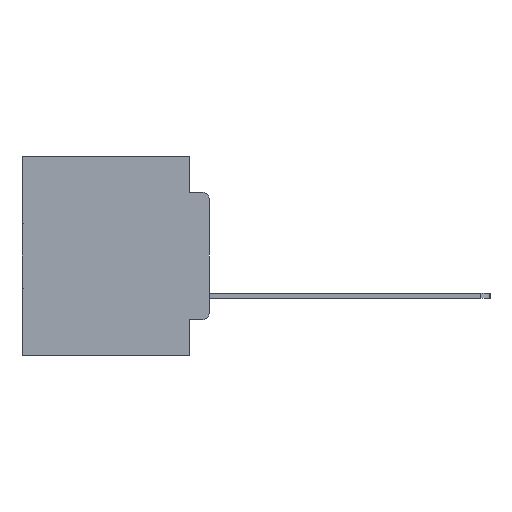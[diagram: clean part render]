
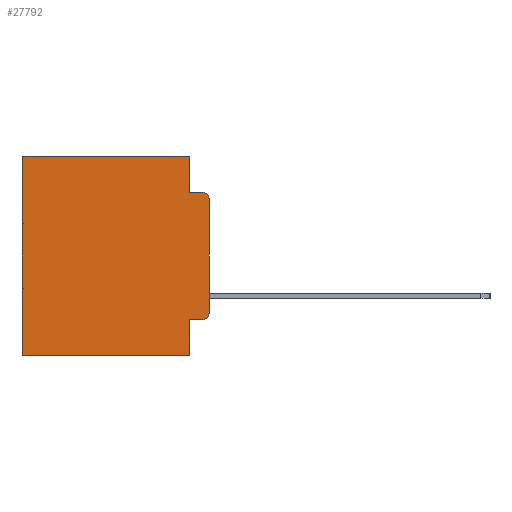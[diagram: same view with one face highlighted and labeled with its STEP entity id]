
A CAD part, left-side view. The second image highlights one B-rep face of the part: STEP entity #27792.
In plain terms, the highlighted planar face has unit normal (-1, 0, 0).
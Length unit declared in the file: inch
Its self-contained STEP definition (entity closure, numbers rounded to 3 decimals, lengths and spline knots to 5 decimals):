
#105 = CARTESIAN_POINT ( 'NONE',  ( 0.298, 0.051, -0.0885 ) ) ;
#163 = VERTEX_POINT ( 'NONE', #20120 ) ;
#319 = VECTOR ( 'NONE', #24453, 39.37008 ) ;
#674 = EDGE_CURVE ( 'NONE', #4658, #4760, #12150, .T. ) ;
#848 = EDGE_LOOP ( 'NONE', ( #5923, #24741, #1097, #13760, #1860, #26917, #8939, #9683, #4096, #4851 ) ) ;
#1097 = ORIENTED_EDGE ( 'NONE', *, *, #29660, .F. ) ;
#1477 = DIRECTION ( 'NONE',  ( 0., 0., -1. ) ) ;
#1490 = VECTOR ( 'NONE', #2249, 39.37008 ) ;
#1860 = ORIENTED_EDGE ( 'NONE', *, *, #14355, .T. ) ;
#2159 = LINE ( 'NONE', #6269, #8470 ) ;
#2249 = DIRECTION ( 'NONE',  ( 0., 0., -1. ) ) ;
#2756 = VECTOR ( 'NONE', #5356, 39.37008 ) ;
#3791 = CARTESIAN_POINT ( 'NONE',  ( 0.298, 0., 0. ) ) ;
#3893 = PLANE ( 'NONE',  #24555 ) ;
#4096 = ORIENTED_EDGE ( 'NONE', *, *, #17200, .T. ) ;
#4294 = LINE ( 'NONE', #7928, #28561 ) ;
#4658 = VERTEX_POINT ( 'NONE', #11114 ) ;
#4760 = VERTEX_POINT ( 'NONE', #12984 ) ;
#4802 = VERTEX_POINT ( 'NONE', #10526 ) ;
#4851 = ORIENTED_EDGE ( 'NONE', *, *, #15642, .T. ) ;
#4865 = LINE ( 'NONE', #7192, #22944 ) ;
#5356 = DIRECTION ( 'NONE',  ( 0., 0., -1. ) ) ;
#5888 = VERTEX_POINT ( 'NONE', #105 ) ;
#5923 = ORIENTED_EDGE ( 'NONE', *, *, #8674, .F. ) ;
#5933 = LINE ( 'NONE', #7991, #319 ) ;
#6269 = CARTESIAN_POINT ( 'NONE',  ( 0.298, 0.051, -0.0885 ) ) ;
#6413 = CARTESIAN_POINT ( 'NONE',  ( 0.298, 0.051, -0.5 ) ) ;
#7025 = LINE ( 'NONE', #18140, #18858 ) ;
#7192 = CARTESIAN_POINT ( 'NONE',  ( 0.298, 0., -0.5 ) ) ;
#7752 = CARTESIAN_POINT ( 'NONE',  ( 0.298, 0.473, 0. ) ) ;
#7928 = CARTESIAN_POINT ( 'NONE',  ( 0.298, 0.051, 0. ) ) ;
#7991 = CARTESIAN_POINT ( 'NONE',  ( 0.298, 0., 0. ) ) ;
#8470 = VECTOR ( 'NONE', #18075, 39.37008 ) ;
#8674 = EDGE_CURVE ( 'NONE', #4658, #16217, #20379, .T. ) ;
#8939 = ORIENTED_EDGE ( 'NONE', *, *, #15885, .F. ) ;
#9683 = ORIENTED_EDGE ( 'NONE', *, *, #18784, .F. ) ;
#9868 = VERTEX_POINT ( 'NONE', #25690 ) ;
#10426 = VECTOR ( 'NONE', #21633, 39.37008 ) ;
#10526 = CARTESIAN_POINT ( 'NONE',  ( 0.298, 0.02, -0.4115 ) ) ;
#11061 = DIRECTION ( 'NONE',  ( 0., 0., -1. ) ) ;
#11114 = CARTESIAN_POINT ( 'NONE',  ( 0.298, 0., -0.1085 ) ) ;
#12150 = CIRCLE ( 'NONE', #23148, 0.02 ) ;
#12770 = CARTESIAN_POINT ( 'NONE',  ( 0.298, 0.051, -0.4115 ) ) ;
#12984 = CARTESIAN_POINT ( 'NONE',  ( 0.298, 0.02, -0.0885 ) ) ;
#13760 = ORIENTED_EDGE ( 'NONE', *, *, #28138, .F. ) ;
#14023 = CARTESIAN_POINT ( 'NONE',  ( 0.298, 0.473, 0. ) ) ;
#14355 = EDGE_CURVE ( 'NONE', #163, #23716, #5933, .T. ) ;
#15642 = EDGE_CURVE ( 'NONE', #4802, #16217, #24791, .T. ) ;
#15712 = DIRECTION ( 'NONE',  ( -1., 0., 0. ) ) ;
#15885 = EDGE_CURVE ( 'NONE', #29084, #9868, #4865, .T. ) ;
#16217 = VERTEX_POINT ( 'NONE', #24859 ) ;
#16486 = CARTESIAN_POINT ( 'NONE',  ( 0.298, 0., 0. ) ) ;
#17200 = EDGE_CURVE ( 'NONE', #26713, #4802, #7025, .T. ) ;
#18075 = DIRECTION ( 'NONE',  ( 0., -1., 0. ) ) ;
#18140 = CARTESIAN_POINT ( 'NONE',  ( 0.298, 0.051, -0.4115 ) ) ;
#18586 = FACE_OUTER_BOUND ( 'NONE', #848, .T. ) ;
#18784 = EDGE_CURVE ( 'NONE', #26713, #29084, #4294, .T. ) ;
#18858 = VECTOR ( 'NONE', #22830, 39.37008 ) ;
#18974 = DIRECTION ( 'NONE',  ( 0., 1., 0. ) ) ;
#19410 = CARTESIAN_POINT ( 'NONE',  ( 0.298, 0.051, 0. ) ) ;
#19712 = DIRECTION ( 'NONE',  ( 0., 0., -1. ) ) ;
#20120 = CARTESIAN_POINT ( 'NONE',  ( 0.298, 0.051, 0. ) ) ;
#20347 = EDGE_CURVE ( 'NONE', #23716, #9868, #27803, .T. ) ;
#20379 = LINE ( 'NONE', #16486, #1490 ) ;
#21633 = DIRECTION ( 'NONE',  ( 0., 0., -1. ) ) ;
#21667 = AXIS2_PLACEMENT_3D ( 'NONE', #29629, #15712, #1477 ) ;
#22830 = DIRECTION ( 'NONE',  ( 0., -1., 0. ) ) ;
#22944 = VECTOR ( 'NONE', #18974, 39.37008 ) ;
#23148 = AXIS2_PLACEMENT_3D ( 'NONE', #24480, #27098, #27067 ) ;
#23716 = VERTEX_POINT ( 'NONE', #14023 ) ;
#24453 = DIRECTION ( 'NONE',  ( 0., 1., 0. ) ) ;
#24480 = CARTESIAN_POINT ( 'NONE',  ( 0.298, 0.02, -0.1085 ) ) ;
#24555 = AXIS2_PLACEMENT_3D ( 'NONE', #3791, #25134, #11061 ) ;
#24741 = ORIENTED_EDGE ( 'NONE', *, *, #674, .T. ) ;
#24791 = CIRCLE ( 'NONE', #21667, 0.02 ) ;
#24859 = CARTESIAN_POINT ( 'NONE',  ( 0.298, 0., -0.3915 ) ) ;
#25134 = DIRECTION ( 'NONE',  ( 1., 0., 0. ) ) ;
#25690 = CARTESIAN_POINT ( 'NONE',  ( 0.298, 0.473, -0.5 ) ) ;
#26713 = VERTEX_POINT ( 'NONE', #12770 ) ;
#26917 = ORIENTED_EDGE ( 'NONE', *, *, #20347, .T. ) ;
#27067 = DIRECTION ( 'NONE',  ( 0., 0., -1. ) ) ;
#27098 = DIRECTION ( 'NONE',  ( -1., 0., 0. ) ) ;
#27792 = ADVANCED_FACE ( 'NONE', ( #18586 ), #3893, .F. ) ;
#27803 = LINE ( 'NONE', #7752, #2756 ) ;
#28138 = EDGE_CURVE ( 'NONE', #163, #5888, #28389, .T. ) ;
#28389 = LINE ( 'NONE', #19410, #10426 ) ;
#28561 = VECTOR ( 'NONE', #19712, 39.37008 ) ;
#29084 = VERTEX_POINT ( 'NONE', #6413 ) ;
#29629 = CARTESIAN_POINT ( 'NONE',  ( 0.298, 0.02, -0.3915 ) ) ;
#29660 = EDGE_CURVE ( 'NONE', #5888, #4760, #2159, .T. ) ;
